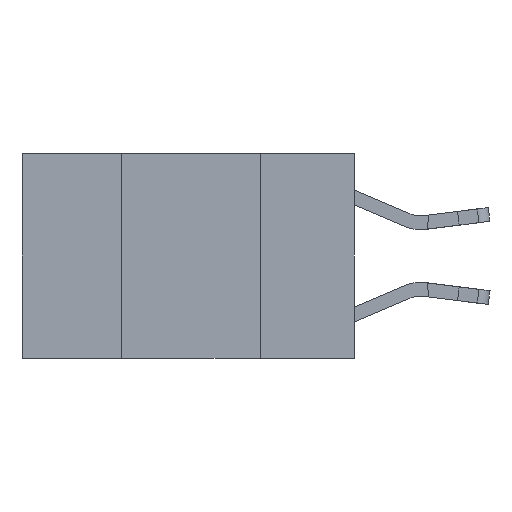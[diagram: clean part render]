
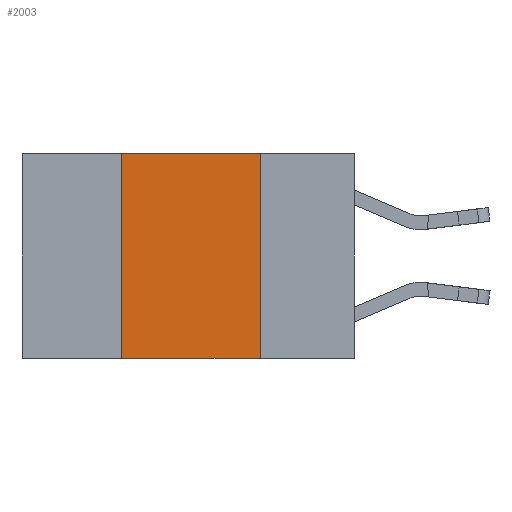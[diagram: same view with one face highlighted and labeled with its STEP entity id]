
A CAD part, left-side view. The second image highlights one B-rep face of the part: STEP entity #2003.
In plain terms, the highlighted planar face has unit normal (-1, 0, 0).
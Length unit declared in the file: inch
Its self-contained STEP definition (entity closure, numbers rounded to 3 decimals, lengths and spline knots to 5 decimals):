
#681 = DIRECTION ( 'NONE',  ( 0., -1., 0. ) ) ;
#1064 = DIRECTION ( 'NONE',  ( 0., 0., -1. ) ) ;
#1441 = CARTESIAN_POINT ( 'NONE',  ( 0., 0.42, 0. ) ) ;
#1599 = CARTESIAN_POINT ( 'NONE',  ( 0., 0.6, 0. ) ) ;
#1678 = EDGE_CURVE ( 'NONE', #5359, #6874, #5334, .T. ) ;
#2003 = ADVANCED_FACE ( 'NONE', ( #9755 ), #8912, .F. ) ;
#2106 = LINE ( 'NONE', #9068, #13258 ) ;
#2488 = DIRECTION ( 'NONE',  ( 0., 0., 1. ) ) ;
#2644 = DIRECTION ( 'NONE',  ( 1., 0., 0. ) ) ;
#2822 = VECTOR ( 'NONE', #2488, 39.37008 ) ;
#2999 = CARTESIAN_POINT ( 'NONE',  ( 0., 0.17, -0.37 ) ) ;
#5112 = EDGE_CURVE ( 'NONE', #12624, #6874, #6840, .T. ) ;
#5182 = ORIENTED_EDGE ( 'NONE', *, *, #10324, .F. ) ;
#5334 = LINE ( 'NONE', #8357, #11219 ) ;
#5359 = VERTEX_POINT ( 'NONE', #6616 ) ;
#5599 = LINE ( 'NONE', #1441, #2822 ) ;
#6616 = CARTESIAN_POINT ( 'NONE',  ( 0., 0.17, 0. ) ) ;
#6840 = LINE ( 'NONE', #7269, #11725 ) ;
#6874 = VERTEX_POINT ( 'NONE', #2999 ) ;
#7009 = ORIENTED_EDGE ( 'NONE', *, *, #1678, .F. ) ;
#7269 = CARTESIAN_POINT ( 'NONE',  ( 0., 0.6, -0.37 ) ) ;
#7712 = EDGE_CURVE ( 'NONE', #12624, #12133, #5599, .T. ) ;
#8202 = EDGE_LOOP ( 'NONE', ( #7009, #5182, #11068, #9291 ) ) ;
#8301 = DIRECTION ( 'NONE',  ( 0., -1., 0. ) ) ;
#8357 = CARTESIAN_POINT ( 'NONE',  ( 0., 0.17, 0. ) ) ;
#8912 = PLANE ( 'NONE',  #10052 ) ;
#9068 = CARTESIAN_POINT ( 'NONE',  ( 0., 0.6, 0. ) ) ;
#9291 = ORIENTED_EDGE ( 'NONE', *, *, #5112, .T. ) ;
#9755 = FACE_OUTER_BOUND ( 'NONE', #8202, .T. ) ;
#9968 = DIRECTION ( 'NONE',  ( 0., 0., -1. ) ) ;
#10052 = AXIS2_PLACEMENT_3D ( 'NONE', #1599, #2644, #9968 ) ;
#10324 = EDGE_CURVE ( 'NONE', #12133, #5359, #2106, .T. ) ;
#11068 = ORIENTED_EDGE ( 'NONE', *, *, #7712, .F. ) ;
#11219 = VECTOR ( 'NONE', #1064, 39.37008 ) ;
#11238 = CARTESIAN_POINT ( 'NONE',  ( 0., 0.42, -0.37 ) ) ;
#11725 = VECTOR ( 'NONE', #8301, 39.37008 ) ;
#12133 = VERTEX_POINT ( 'NONE', #12913 ) ;
#12624 = VERTEX_POINT ( 'NONE', #11238 ) ;
#12913 = CARTESIAN_POINT ( 'NONE',  ( 0., 0.42, 0. ) ) ;
#13258 = VECTOR ( 'NONE', #681, 39.37008 ) ;
